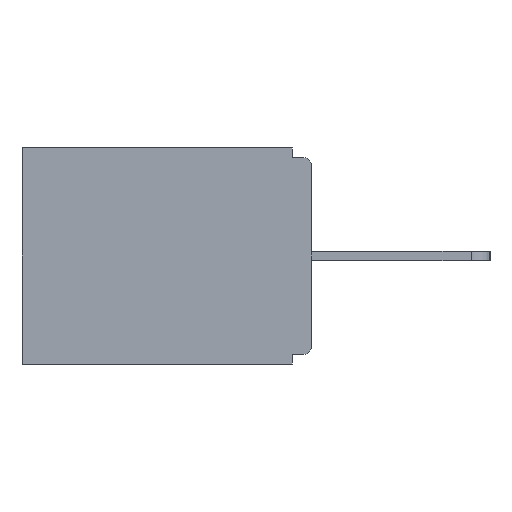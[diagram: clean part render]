
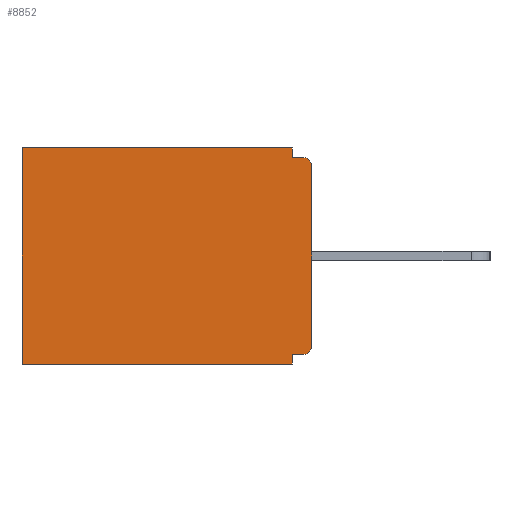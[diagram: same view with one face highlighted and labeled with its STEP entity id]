
A CAD part, left-side view. The second image highlights one B-rep face of the part: STEP entity #8852.
In plain terms, the highlighted planar face has unit normal (-1, 0, 0).
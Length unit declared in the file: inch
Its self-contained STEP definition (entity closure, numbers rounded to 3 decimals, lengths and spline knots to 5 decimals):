
#518 = CARTESIAN_POINT ( 'NONE',  ( 0.298, 0.46, 0. ) ) ;
#678 = DIRECTION ( 'NONE',  ( 0., 0., -1. ) ) ;
#764 = VECTOR ( 'NONE', #11176, 39.37008 ) ;
#787 = VERTEX_POINT ( 'NONE', #21183 ) ;
#983 = ORIENTED_EDGE ( 'NONE', *, *, #14139, .T. ) ;
#1634 = ORIENTED_EDGE ( 'NONE', *, *, #19250, .F. ) ;
#2156 = VECTOR ( 'NONE', #18852, 39.37008 ) ;
#2292 = PLANE ( 'NONE',  #17999 ) ;
#2593 = ORIENTED_EDGE ( 'NONE', *, *, #13009, .T. ) ;
#2861 = ORIENTED_EDGE ( 'NONE', *, *, #6376, .F. ) ;
#3344 = CARTESIAN_POINT ( 'NONE',  ( 0.298, 0.015, -0.313 ) ) ;
#4015 = VERTEX_POINT ( 'NONE', #7046 ) ;
#4178 = ORIENTED_EDGE ( 'NONE', *, *, #9623, .T. ) ;
#4184 = LINE ( 'NONE', #18912, #20747 ) ;
#4252 = LINE ( 'NONE', #7915, #14516 ) ;
#4471 = CIRCLE ( 'NONE', #15900, 0.015 ) ;
#4644 = VERTEX_POINT ( 'NONE', #21271 ) ;
#4732 = ORIENTED_EDGE ( 'NONE', *, *, #18640, .F. ) ;
#5418 = CARTESIAN_POINT ( 'NONE',  ( 0.298, 0.031, -0.343 ) ) ;
#5424 = ORIENTED_EDGE ( 'NONE', *, *, #12115, .T. ) ;
#5499 = DIRECTION ( 'NONE',  ( 0., 0., -1. ) ) ;
#5634 = FACE_OUTER_BOUND ( 'NONE', #8483, .T. ) ;
#6376 = EDGE_CURVE ( 'NONE', #16586, #14554, #16882, .T. ) ;
#6590 = CIRCLE ( 'NONE', #18690, 0.015 ) ;
#6777 = ORIENTED_EDGE ( 'NONE', *, *, #10176, .F. ) ;
#6953 = CARTESIAN_POINT ( 'NONE',  ( 0.298, 0.015, -0.03 ) ) ;
#7046 = CARTESIAN_POINT ( 'NONE',  ( 0.298, 0.031, -0.328 ) ) ;
#7353 = CARTESIAN_POINT ( 'NONE',  ( 0.298, 0., -0.328 ) ) ;
#7383 = LINE ( 'NONE', #5418, #2156 ) ;
#7915 = CARTESIAN_POINT ( 'NONE',  ( 0.298, 0., -0.343 ) ) ;
#8141 = VERTEX_POINT ( 'NONE', #15787 ) ;
#8150 = EDGE_CURVE ( 'NONE', #8141, #787, #4184, .T. ) ;
#8471 = DIRECTION ( 'NONE',  ( 0., 0., -1. ) ) ;
#8483 = EDGE_LOOP ( 'NONE', ( #2593, #16042, #6777, #983, #4178, #4732, #12674, #1634, #5424, #2861 ) ) ;
#8817 = VECTOR ( 'NONE', #5499, 39.37008 ) ;
#8852 = ADVANCED_FACE ( 'NONE', ( #5634 ), #2292, .F. ) ;
#9606 = DIRECTION ( 'NONE',  ( -1., 0., 0. ) ) ;
#9623 = EDGE_CURVE ( 'NONE', #21330, #4644, #14473, .T. ) ;
#10176 = EDGE_CURVE ( 'NONE', #19949, #8141, #7383, .T. ) ;
#10264 = CARTESIAN_POINT ( 'NONE',  ( 0.298, 0., 0. ) ) ;
#10701 = DIRECTION ( 'NONE',  ( 1., 0., 0. ) ) ;
#11176 = DIRECTION ( 'NONE',  ( 0., 1., 0. ) ) ;
#12115 = EDGE_CURVE ( 'NONE', #16829, #14554, #4471, .T. ) ;
#12162 = CARTESIAN_POINT ( 'NONE',  ( 0.298, 0.015, -0.328 ) ) ;
#12478 = DIRECTION ( 'NONE',  ( 0., 1., 0. ) ) ;
#12584 = CARTESIAN_POINT ( 'NONE',  ( 0.298, 0., 0. ) ) ;
#12674 = ORIENTED_EDGE ( 'NONE', *, *, #18576, .F. ) ;
#13009 = EDGE_CURVE ( 'NONE', #16586, #787, #6590, .T. ) ;
#13253 = DIRECTION ( 'NONE',  ( -1., 0., 0. ) ) ;
#13518 = LINE ( 'NONE', #7353, #21098 ) ;
#13967 = DIRECTION ( 'NONE',  ( 0., 1., 0. ) ) ;
#14139 = EDGE_CURVE ( 'NONE', #19949, #21330, #21130, .T. ) ;
#14473 = LINE ( 'NONE', #19465, #18720 ) ;
#14516 = VECTOR ( 'NONE', #12478, 39.37008 ) ;
#14554 = VERTEX_POINT ( 'NONE', #19363 ) ;
#14717 = DIRECTION ( 'NONE',  ( 0., 0., -1. ) ) ;
#14851 = CARTESIAN_POINT ( 'NONE',  ( 0.298, 0.031, -0.343 ) ) ;
#15525 = LINE ( 'NONE', #20615, #20405 ) ;
#15787 = CARTESIAN_POINT ( 'NONE',  ( 0.298, 0.031, -0.015 ) ) ;
#15900 = AXIS2_PLACEMENT_3D ( 'NONE', #3344, #9606, #14717 ) ;
#16042 = ORIENTED_EDGE ( 'NONE', *, *, #8150, .F. ) ;
#16093 = CARTESIAN_POINT ( 'NONE',  ( 0.298, 0., -0.03 ) ) ;
#16586 = VERTEX_POINT ( 'NONE', #16093 ) ;
#16829 = VERTEX_POINT ( 'NONE', #12162 ) ;
#16882 = LINE ( 'NONE', #10264, #8817 ) ;
#17124 = CARTESIAN_POINT ( 'NONE',  ( 0.298, 0., 0. ) ) ;
#17295 = DIRECTION ( 'NONE',  ( 0., -1., 0. ) ) ;
#17999 = AXIS2_PLACEMENT_3D ( 'NONE', #17124, #10701, #20349 ) ;
#18576 = EDGE_CURVE ( 'NONE', #4015, #18833, #15525, .T. ) ;
#18640 = EDGE_CURVE ( 'NONE', #18833, #4644, #4252, .T. ) ;
#18690 = AXIS2_PLACEMENT_3D ( 'NONE', #6953, #13253, #8471 ) ;
#18720 = VECTOR ( 'NONE', #21301, 39.37008 ) ;
#18833 = VERTEX_POINT ( 'NONE', #14851 ) ;
#18852 = DIRECTION ( 'NONE',  ( 0., 0., -1. ) ) ;
#18912 = CARTESIAN_POINT ( 'NONE',  ( 0.298, 0., -0.015 ) ) ;
#19250 = EDGE_CURVE ( 'NONE', #16829, #4015, #13518, .T. ) ;
#19363 = CARTESIAN_POINT ( 'NONE',  ( 0.298, 0., -0.313 ) ) ;
#19440 = CARTESIAN_POINT ( 'NONE',  ( 0.298, 0.031, 0. ) ) ;
#19465 = CARTESIAN_POINT ( 'NONE',  ( 0.298, 0.46, 0. ) ) ;
#19949 = VERTEX_POINT ( 'NONE', #19440 ) ;
#20349 = DIRECTION ( 'NONE',  ( 0., 0., -1. ) ) ;
#20405 = VECTOR ( 'NONE', #678, 39.37008 ) ;
#20615 = CARTESIAN_POINT ( 'NONE',  ( 0.298, 0.031, -0.343 ) ) ;
#20747 = VECTOR ( 'NONE', #17295, 39.37008 ) ;
#21098 = VECTOR ( 'NONE', #13967, 39.37008 ) ;
#21130 = LINE ( 'NONE', #12584, #764 ) ;
#21183 = CARTESIAN_POINT ( 'NONE',  ( 0.298, 0.015, -0.015 ) ) ;
#21271 = CARTESIAN_POINT ( 'NONE',  ( 0.298, 0.46, -0.343 ) ) ;
#21301 = DIRECTION ( 'NONE',  ( 0., 0., -1. ) ) ;
#21330 = VERTEX_POINT ( 'NONE', #518 ) ;
